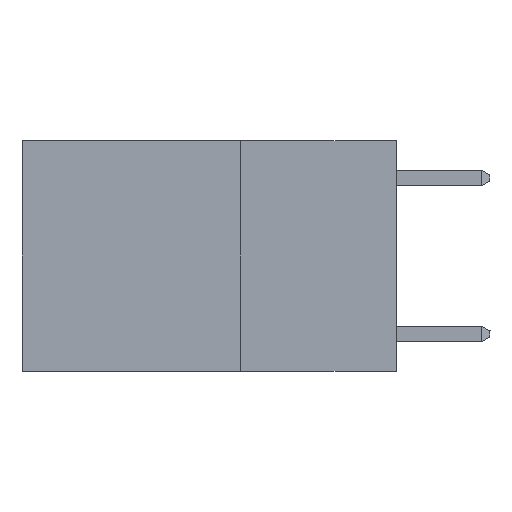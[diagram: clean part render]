
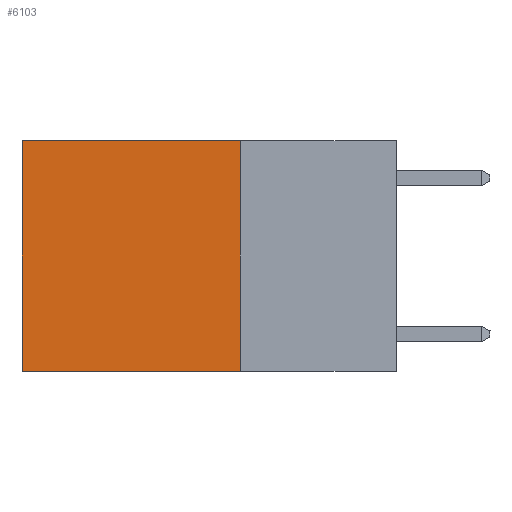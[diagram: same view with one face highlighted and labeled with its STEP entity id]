
A CAD part, left-side view. The second image highlights one B-rep face of the part: STEP entity #6103.
In plain terms, the highlighted planar face has unit normal (-1, 0, 0).
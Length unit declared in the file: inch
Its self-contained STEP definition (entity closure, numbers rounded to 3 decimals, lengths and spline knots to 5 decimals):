
#470 = ORIENTED_EDGE ( 'NONE', *, *, #1989, .T. ) ;
#494 = ORIENTED_EDGE ( 'NONE', *, *, #4717, .F. ) ;
#528 = ORIENTED_EDGE ( 'NONE', *, *, #4778, .F. ) ;
#537 = ORIENTED_EDGE ( 'NONE', *, *, #924, .T. ) ;
#552 = VERTEX_POINT ( 'NONE', #2958 ) ;
#924 = EDGE_CURVE ( 'NONE', #552, #9574, #1827, .T. ) ;
#1148 = CARTESIAN_POINT ( 'NONE',  ( 0.2625, 0.25, 0. ) ) ;
#1392 = FACE_OUTER_BOUND ( 'NONE', #3484, .T. ) ;
#1827 = LINE ( 'NONE', #5421, #3591 ) ;
#1855 = DIRECTION ( 'NONE',  ( 0., 0., -1. ) ) ;
#1942 = VECTOR ( 'NONE', #6361, 39.37008 ) ;
#1989 = EDGE_CURVE ( 'NONE', #9574, #4012, #8895, .T. ) ;
#2035 = DIRECTION ( 'NONE',  ( 0., 0., -1. ) ) ;
#2455 = VERTEX_POINT ( 'NONE', #4648 ) ;
#2793 = DIRECTION ( 'NONE',  ( 0., 1., 0. ) ) ;
#2958 = CARTESIAN_POINT ( 'NONE',  ( 0.2625, 0.25, 0. ) ) ;
#3484 = EDGE_LOOP ( 'NONE', ( #470, #494, #528, #537 ) ) ;
#3591 = VECTOR ( 'NONE', #2793, 39.37008 ) ;
#4012 = VERTEX_POINT ( 'NONE', #5620 ) ;
#4590 = VECTOR ( 'NONE', #1855, 39.37008 ) ;
#4648 = CARTESIAN_POINT ( 'NONE',  ( 0.2625, 0.25, -0.37 ) ) ;
#4697 = CARTESIAN_POINT ( 'NONE',  ( 0.2625, 0.6, 0. ) ) ;
#4717 = EDGE_CURVE ( 'NONE', #2455, #4012, #5363, .T. ) ;
#4778 = EDGE_CURVE ( 'NONE', #552, #2455, #8720, .T. ) ;
#5363 = LINE ( 'NONE', #10859, #7286 ) ;
#5421 = CARTESIAN_POINT ( 'NONE',  ( 0.2625, 0.25, 0. ) ) ;
#5459 = CARTESIAN_POINT ( 'NONE',  ( 0.2625, 0.6, 0. ) ) ;
#5620 = CARTESIAN_POINT ( 'NONE',  ( 0.2625, 0.6, -0.37 ) ) ;
#6103 = ADVANCED_FACE ( 'NONE', ( #1392 ), #6247, .F. ) ;
#6247 = PLANE ( 'NONE',  #7200 ) ;
#6361 = DIRECTION ( 'NONE',  ( 0., 0., -1. ) ) ;
#6840 = DIRECTION ( 'NONE',  ( 0., 1., 0. ) ) ;
#7062 = DIRECTION ( 'NONE',  ( 1., 0., 0. ) ) ;
#7200 = AXIS2_PLACEMENT_3D ( 'NONE', #1148, #7062, #2035 ) ;
#7286 = VECTOR ( 'NONE', #6840, 39.37008 ) ;
#8720 = LINE ( 'NONE', #10183, #4590 ) ;
#8895 = LINE ( 'NONE', #4697, #1942 ) ;
#9574 = VERTEX_POINT ( 'NONE', #5459 ) ;
#10183 = CARTESIAN_POINT ( 'NONE',  ( 0.2625, 0.25, 0. ) ) ;
#10859 = CARTESIAN_POINT ( 'NONE',  ( 0.2625, 0.25, -0.37 ) ) ;
